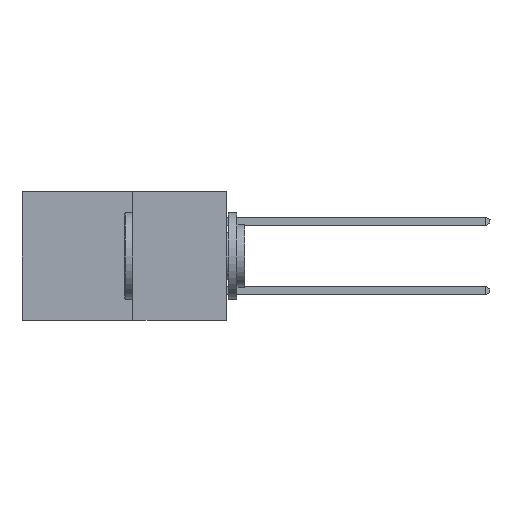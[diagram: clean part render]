
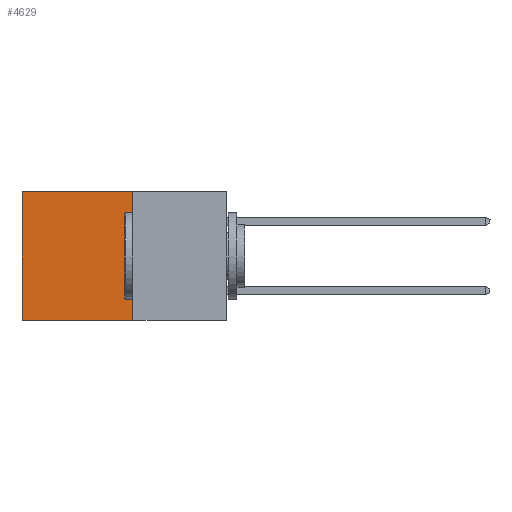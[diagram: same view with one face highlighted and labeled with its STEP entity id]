
A CAD part, left-side view. The second image highlights one B-rep face of the part: STEP entity #4629.
In plain terms, the highlighted planar face has unit normal (-1, 0, 0).
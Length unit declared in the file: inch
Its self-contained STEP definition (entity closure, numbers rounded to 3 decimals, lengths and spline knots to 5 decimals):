
#787 = ORIENTED_EDGE ( 'NONE', *, *, #10563, .F. ) ;
#2194 = CARTESIAN_POINT ( 'NONE',  ( 0.277, 0.27, -0.37 ) ) ;
#3064 = DIRECTION ( 'NONE',  ( 0., 1., 0. ) ) ;
#3927 = EDGE_CURVE ( 'NONE', #17510, #13840, #5673, .T. ) ;
#4322 = DIRECTION ( 'NONE',  ( 0., 0., -1. ) ) ;
#4629 = ADVANCED_FACE ( 'NONE', ( #4640 ), #11886, .F. ) ;
#4640 = FACE_OUTER_BOUND ( 'NONE', #18067, .T. ) ;
#4700 = LINE ( 'NONE', #20065, #15034 ) ;
#4932 = VERTEX_POINT ( 'NONE', #5885 ) ;
#5353 = CARTESIAN_POINT ( 'NONE',  ( 0.277, 0.27, 0. ) ) ;
#5673 = LINE ( 'NONE', #17381, #21314 ) ;
#5797 = EDGE_CURVE ( 'NONE', #4932, #17510, #26256, .T. ) ;
#5885 = CARTESIAN_POINT ( 'NONE',  ( 0.277, 0.27, 0. ) ) ;
#6064 = ORIENTED_EDGE ( 'NONE', *, *, #3927, .T. ) ;
#9869 = VECTOR ( 'NONE', #4322, 39.37008 ) ;
#10563 = EDGE_CURVE ( 'NONE', #4932, #13087, #20079, .T. ) ;
#10988 = CARTESIAN_POINT ( 'NONE',  ( 0.277, 0.59, 0. ) ) ;
#11026 = DIRECTION ( 'NONE',  ( 0., 0., -1. ) ) ;
#11095 = DIRECTION ( 'NONE',  ( 1., 0., 0. ) ) ;
#11886 = PLANE ( 'NONE',  #25862 ) ;
#11960 = DIRECTION ( 'NONE',  ( 0., 1., 0. ) ) ;
#13087 = VERTEX_POINT ( 'NONE', #18061 ) ;
#13840 = VERTEX_POINT ( 'NONE', #22292 ) ;
#15034 = VECTOR ( 'NONE', #11960, 39.37008 ) ;
#15540 = CARTESIAN_POINT ( 'NONE',  ( 0.277, 0.27, -0.37 ) ) ;
#17381 = CARTESIAN_POINT ( 'NONE',  ( 0.277, 0.59, -0.37 ) ) ;
#17510 = VERTEX_POINT ( 'NONE', #10988 ) ;
#17968 = ORIENTED_EDGE ( 'NONE', *, *, #5797, .T. ) ;
#18061 = CARTESIAN_POINT ( 'NONE',  ( 0.277, 0.27, -0.37 ) ) ;
#18067 = EDGE_LOOP ( 'NONE', ( #6064, #19539, #787, #17968 ) ) ;
#19247 = DIRECTION ( 'NONE',  ( 0., 0., -1. ) ) ;
#19539 = ORIENTED_EDGE ( 'NONE', *, *, #19899, .F. ) ;
#19899 = EDGE_CURVE ( 'NONE', #13087, #13840, #4700, .T. ) ;
#20065 = CARTESIAN_POINT ( 'NONE',  ( 0.277, 0.27, -0.37 ) ) ;
#20079 = LINE ( 'NONE', #2194, #9869 ) ;
#20931 = VECTOR ( 'NONE', #3064, 39.37008 ) ;
#21314 = VECTOR ( 'NONE', #19247, 39.37008 ) ;
#22292 = CARTESIAN_POINT ( 'NONE',  ( 0.277, 0.59, -0.37 ) ) ;
#25862 = AXIS2_PLACEMENT_3D ( 'NONE', #15540, #11095, #11026 ) ;
#26256 = LINE ( 'NONE', #5353, #20931 ) ;
